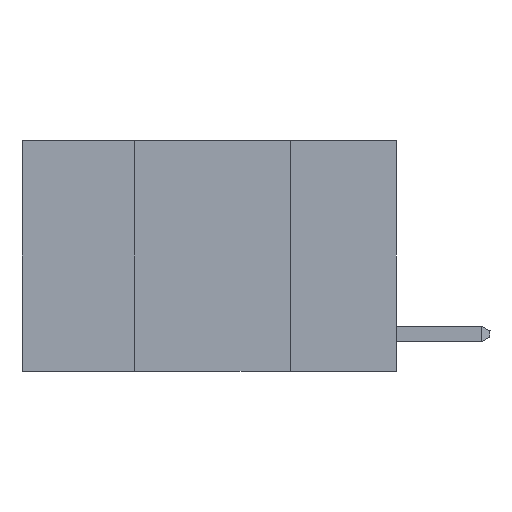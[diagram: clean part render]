
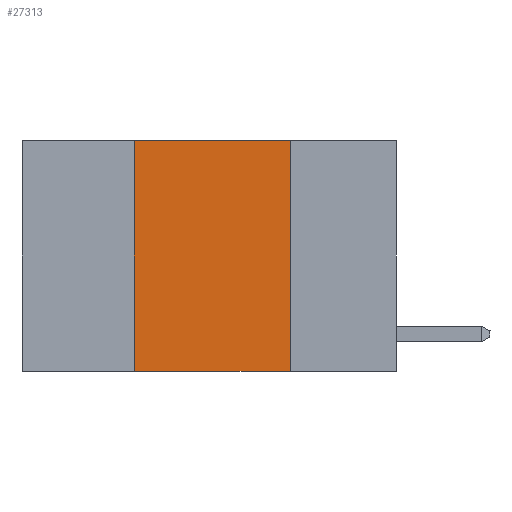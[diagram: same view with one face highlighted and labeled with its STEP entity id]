
A CAD part, left-side view. The second image highlights one B-rep face of the part: STEP entity #27313.
In plain terms, the highlighted planar face has unit normal (-1, 0, 0).
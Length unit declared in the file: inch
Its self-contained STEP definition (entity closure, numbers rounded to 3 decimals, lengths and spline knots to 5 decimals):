
#814 = CARTESIAN_POINT ( 'NONE',  ( 0., 0.42, -0.37 ) ) ;
#1314 = DIRECTION ( 'NONE',  ( 0., -1., 0. ) ) ;
#1438 = CARTESIAN_POINT ( 'NONE',  ( 0., 0.17, 0. ) ) ;
#2972 = VECTOR ( 'NONE', #25764, 39.37008 ) ;
#4607 = VERTEX_POINT ( 'NONE', #6587 ) ;
#5771 = VERTEX_POINT ( 'NONE', #10389 ) ;
#5818 = EDGE_CURVE ( 'NONE', #15156, #5771, #17969, .T. ) ;
#6587 = CARTESIAN_POINT ( 'NONE',  ( 0., 0.17, -0.37 ) ) ;
#6980 = ORIENTED_EDGE ( 'NONE', *, *, #26742, .T. ) ;
#7477 = EDGE_CURVE ( 'NONE', #12318, #15156, #7539, .T. ) ;
#7539 = LINE ( 'NONE', #14593, #18565 ) ;
#7839 = CARTESIAN_POINT ( 'NONE',  ( 0., 0.6, -0.37 ) ) ;
#8752 = LINE ( 'NONE', #1438, #2972 ) ;
#9166 = DIRECTION ( 'NONE',  ( 1., 0., 0. ) ) ;
#10389 = CARTESIAN_POINT ( 'NONE',  ( 0., 0.17, 0. ) ) ;
#10579 = DIRECTION ( 'NONE',  ( 0., -1., 0. ) ) ;
#10698 = ORIENTED_EDGE ( 'NONE', *, *, #7477, .F. ) ;
#11287 = PLANE ( 'NONE',  #26233 ) ;
#12318 = VERTEX_POINT ( 'NONE', #814 ) ;
#14472 = ORIENTED_EDGE ( 'NONE', *, *, #22798, .F. ) ;
#14593 = CARTESIAN_POINT ( 'NONE',  ( 0., 0.42, 0. ) ) ;
#14672 = VECTOR ( 'NONE', #1314, 39.37008 ) ;
#15156 = VERTEX_POINT ( 'NONE', #19575 ) ;
#17063 = FACE_OUTER_BOUND ( 'NONE', #25539, .T. ) ;
#17949 = CARTESIAN_POINT ( 'NONE',  ( 0., 0.6, 0. ) ) ;
#17969 = LINE ( 'NONE', #23863, #25292 ) ;
#18565 = VECTOR ( 'NONE', #28026, 39.37008 ) ;
#19575 = CARTESIAN_POINT ( 'NONE',  ( 0., 0.42, 0. ) ) ;
#22798 = EDGE_CURVE ( 'NONE', #5771, #4607, #8752, .T. ) ;
#23863 = CARTESIAN_POINT ( 'NONE',  ( 0., 0.6, 0. ) ) ;
#24667 = DIRECTION ( 'NONE',  ( 0., 0., -1. ) ) ;
#25292 = VECTOR ( 'NONE', #10579, 39.37008 ) ;
#25539 = EDGE_LOOP ( 'NONE', ( #14472, #26327, #10698, #6980 ) ) ;
#25764 = DIRECTION ( 'NONE',  ( 0., 0., -1. ) ) ;
#26233 = AXIS2_PLACEMENT_3D ( 'NONE', #17949, #9166, #24667 ) ;
#26327 = ORIENTED_EDGE ( 'NONE', *, *, #5818, .F. ) ;
#26527 = LINE ( 'NONE', #7839, #14672 ) ;
#26742 = EDGE_CURVE ( 'NONE', #12318, #4607, #26527, .T. ) ;
#27313 = ADVANCED_FACE ( 'NONE', ( #17063 ), #11287, .F. ) ;
#28026 = DIRECTION ( 'NONE',  ( 0., 0., 1. ) ) ;
